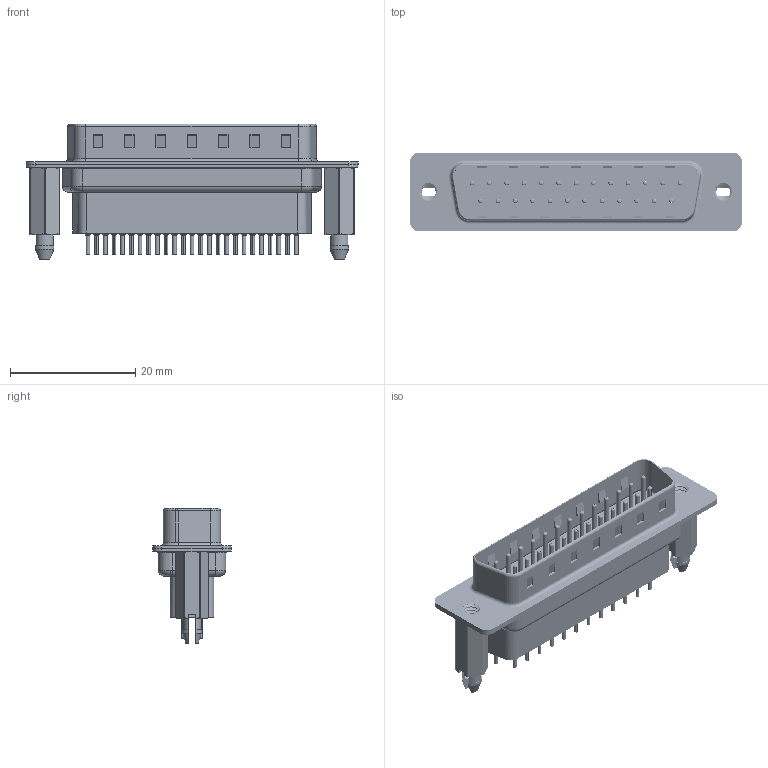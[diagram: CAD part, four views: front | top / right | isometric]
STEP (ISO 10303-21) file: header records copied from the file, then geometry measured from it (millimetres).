
FILE_DESCRIPTION (( 'STEP AP203' ), '1' );
FILE_NAME ('627-025-621-276.STEP', '2020-07-14T22:55:23', ( '' ), ( '' ), 'SwSTEP 2.0', 'SolidWorks 2020', '' );
FILE_SCHEMA (( 'CONFIG_CONTROL_DESIGN' ));
Length unit declared in the file: millimetre
Products named in the file (7): 627 Contact Row 2_21H; 627 Contact Row 1_21H; 627 Shell Rear_25 Contacts; 627 4-40 Threaded Boardlock_HP; 627 Shell Front_25 Contacts; 627 Housing_25 HP; 627-025-621-276
Assembly tree (30 placements, depth 2):
  627-025-621-276
    627 Housing_25 HP
    627 Shell Front_25 Contacts
    627 Shell Rear_25 Contacts
    627 Contact Row 1_21H  x13
    627 Contact Row 2_21H  x12
    627 4-40 Threaded Boardlock_HP  x2
Bounding box: 53 x 12.6 x 21.7 mm (x, y, z)
Volume: 4049.3 mm3; surface area: 10359.5 mm2
Topology: 30 solids, 30 shells, 2940 faces, 7659 edges, 4813 vertices
Faces by surface type: cylinder 1130, plane 803, torus 731, cone 266, bspline 10
Entity records: 28757 total; most frequent: CARTESIAN_POINT 8037, DIRECTION 4248, ORIENTED_EDGE 3944, EDGE_CURVE 1972, AXIS2_PLACEMENT_3D 1665, VERTEX_POINT 1262, EDGE_LOOP 930, VECTOR 918
